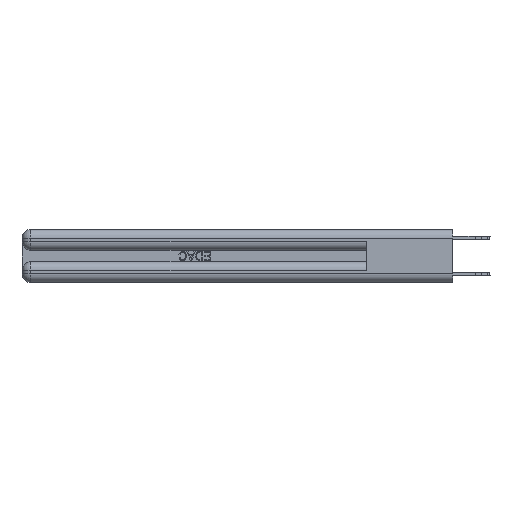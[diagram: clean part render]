
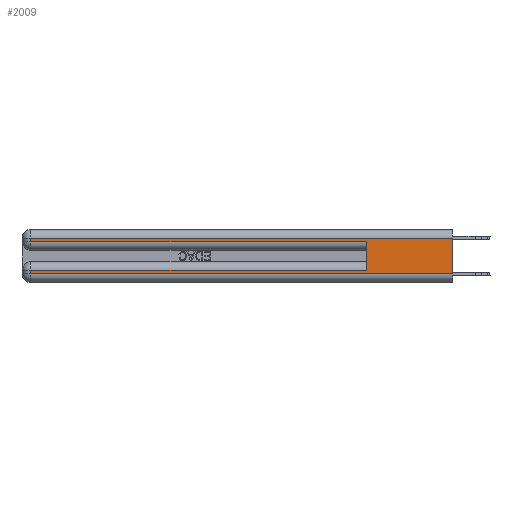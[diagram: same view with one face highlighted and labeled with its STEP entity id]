
A CAD part, left-side view. The second image highlights one B-rep face of the part: STEP entity #2009.
In plain terms, the highlighted planar face has unit normal (-1, 0, 0).
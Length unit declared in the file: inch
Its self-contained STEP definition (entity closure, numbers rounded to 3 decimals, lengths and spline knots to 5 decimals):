
#419 = DIRECTION ( 'NONE',  ( 0., -1., 0. ) ) ;
#601 = CARTESIAN_POINT ( 'NONE',  ( 0., 0.6, 0.145 ) ) ;
#887 = EDGE_CURVE ( 'NONE', #14613, #18202, #2787, .T. ) ;
#2009 = ADVANCED_FACE ( 'NONE', ( #16705 ), #7658, .F. ) ;
#2191 = VERTEX_POINT ( 'NONE', #25613 ) ;
#2553 = CARTESIAN_POINT ( 'NONE',  ( 0., 0., 0.31 ) ) ;
#2694 = DIRECTION ( 'NONE',  ( 1., 0., 0. ) ) ;
#2787 = LINE ( 'NONE', #24042, #11009 ) ;
#3097 = EDGE_CURVE ( 'NONE', #4839, #2191, #28609, .T. ) ;
#3600 = DIRECTION ( 'NONE',  ( 0., 1., 0. ) ) ;
#3895 = VERTEX_POINT ( 'NONE', #10652 ) ;
#4713 = ORIENTED_EDGE ( 'NONE', *, *, #27850, .F. ) ;
#4839 = VERTEX_POINT ( 'NONE', #28739 ) ;
#4951 = DIRECTION ( 'NONE',  ( 0., -1., 0. ) ) ;
#4956 = VECTOR ( 'NONE', #19300, 39.37008 ) ;
#6316 = ORIENTED_EDGE ( 'NONE', *, *, #7600, .T. ) ;
#6402 = VECTOR ( 'NONE', #3600, 39.37008 ) ;
#6615 = ORIENTED_EDGE ( 'NONE', *, *, #887, .T. ) ;
#7550 = CARTESIAN_POINT ( 'NONE',  ( 0., 2.94, 0.06 ) ) ;
#7584 = CARTESIAN_POINT ( 'NONE',  ( 0., 0., 0.285 ) ) ;
#7600 = EDGE_CURVE ( 'NONE', #18202, #2191, #26032, .T. ) ;
#7658 = PLANE ( 'NONE',  #19284 ) ;
#9122 = ORIENTED_EDGE ( 'NONE', *, *, #29350, .T. ) ;
#9387 = EDGE_CURVE ( 'NONE', #18262, #10302, #9998, .T. ) ;
#9432 = ORIENTED_EDGE ( 'NONE', *, *, #9387, .T. ) ;
#9739 = CARTESIAN_POINT ( 'NONE',  ( 0., 0., 0.085 ) ) ;
#9763 = EDGE_LOOP ( 'NONE', ( #4713, #9122, #6615, #6316, #11050, #30026, #30335, #9432 ) ) ;
#9846 = DIRECTION ( 'NONE',  ( 0., 0., 1. ) ) ;
#9998 = LINE ( 'NONE', #14310, #16413 ) ;
#10270 = EDGE_CURVE ( 'NONE', #3895, #18262, #25790, .T. ) ;
#10302 = VERTEX_POINT ( 'NONE', #23773 ) ;
#10652 = CARTESIAN_POINT ( 'NONE',  ( 0., 2.94, 0.085 ) ) ;
#11009 = VECTOR ( 'NONE', #16814, 39.37008 ) ;
#11050 = ORIENTED_EDGE ( 'NONE', *, *, #3097, .F. ) ;
#12298 = CARTESIAN_POINT ( 'NONE',  ( 0., 2.94, 0.285 ) ) ;
#14310 = CARTESIAN_POINT ( 'NONE',  ( 0., 0., 0.06 ) ) ;
#14613 = VERTEX_POINT ( 'NONE', #26465 ) ;
#16413 = VECTOR ( 'NONE', #419, 39.37008 ) ;
#16519 = LINE ( 'NONE', #9739, #16885 ) ;
#16705 = FACE_OUTER_BOUND ( 'NONE', #9763, .T. ) ;
#16814 = DIRECTION ( 'NONE',  ( 0., 0., -1. ) ) ;
#16885 = VECTOR ( 'NONE', #28043, 39.37008 ) ;
#17024 = CARTESIAN_POINT ( 'NONE',  ( 0., 0., 0.37 ) ) ;
#17330 = CARTESIAN_POINT ( 'NONE',  ( 0., 0., 0.31 ) ) ;
#18114 = LINE ( 'NONE', #27500, #23672 ) ;
#18202 = VERTEX_POINT ( 'NONE', #12298 ) ;
#18262 = VERTEX_POINT ( 'NONE', #7550 ) ;
#19284 = AXIS2_PLACEMENT_3D ( 'NONE', #17024, #2694, #21484 ) ;
#19300 = DIRECTION ( 'NONE',  ( 0., 0., -1. ) ) ;
#20265 = DIRECTION ( 'NONE',  ( 0., 0., -1. ) ) ;
#20575 = EDGE_CURVE ( 'NONE', #4839, #3895, #16519, .T. ) ;
#21484 = DIRECTION ( 'NONE',  ( 0., 0., -1. ) ) ;
#22043 = VERTEX_POINT ( 'NONE', #2553 ) ;
#23672 = VECTOR ( 'NONE', #20265, 39.37008 ) ;
#23773 = CARTESIAN_POINT ( 'NONE',  ( 0., 0., 0.06 ) ) ;
#24042 = CARTESIAN_POINT ( 'NONE',  ( 0., 2.94, 0.37 ) ) ;
#25613 = CARTESIAN_POINT ( 'NONE',  ( 0., 0.6, 0.285 ) ) ;
#25790 = LINE ( 'NONE', #28057, #4956 ) ;
#26032 = LINE ( 'NONE', #7584, #28861 ) ;
#26465 = CARTESIAN_POINT ( 'NONE',  ( 0., 2.94, 0.31 ) ) ;
#26877 = LINE ( 'NONE', #17330, #6402 ) ;
#27500 = CARTESIAN_POINT ( 'NONE',  ( 0., 0., 0.37 ) ) ;
#27850 = EDGE_CURVE ( 'NONE', #22043, #10302, #18114, .T. ) ;
#28043 = DIRECTION ( 'NONE',  ( 0., 1., 0. ) ) ;
#28057 = CARTESIAN_POINT ( 'NONE',  ( 0., 2.94, 0.37 ) ) ;
#28220 = VECTOR ( 'NONE', #9846, 39.37008 ) ;
#28609 = LINE ( 'NONE', #601, #28220 ) ;
#28739 = CARTESIAN_POINT ( 'NONE',  ( 0., 0.6, 0.085 ) ) ;
#28861 = VECTOR ( 'NONE', #4951, 39.37008 ) ;
#29350 = EDGE_CURVE ( 'NONE', #22043, #14613, #26877, .T. ) ;
#30026 = ORIENTED_EDGE ( 'NONE', *, *, #20575, .T. ) ;
#30335 = ORIENTED_EDGE ( 'NONE', *, *, #10270, .T. ) ;
